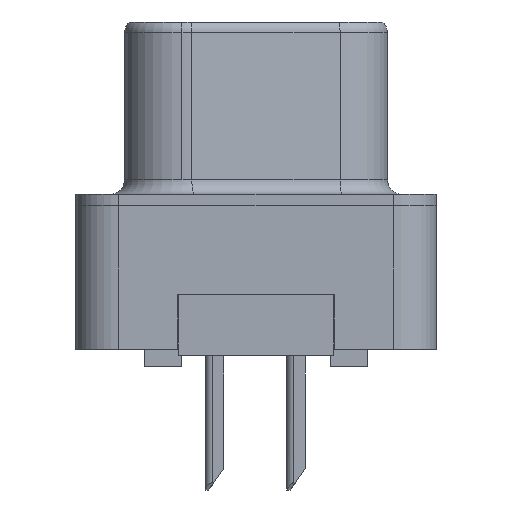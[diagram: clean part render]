
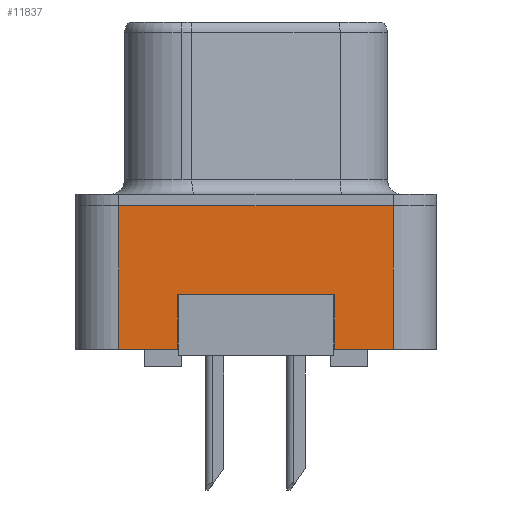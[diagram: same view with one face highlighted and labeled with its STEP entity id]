
A CAD part, left-side view. The second image highlights one B-rep face of the part: STEP entity #11837.
In plain terms, the highlighted planar face has unit normal (-1, 0, 0).
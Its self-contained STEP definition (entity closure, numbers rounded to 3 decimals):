
#8 = LINE ( 'NONE', #12915, #7780 ) ;
#268 = DIRECTION ( 'NONE',  ( 0., 0., 1. ) ) ;
#650 = LINE ( 'NONE', #9021, #14056 ) ;
#804 = CARTESIAN_POINT ( 'NONE',  ( -2.91, 2.75, -5. ) ) ;
#866 = VERTEX_POINT ( 'NONE', #6942 ) ;
#1035 = ORIENTED_EDGE ( 'NONE', *, *, #11643, .F. ) ;
#1530 = VECTOR ( 'NONE', #8417, 1000. ) ;
#1874 = DIRECTION ( 'NONE',  ( 0., -1., 0. ) ) ;
#2149 = ORIENTED_EDGE ( 'NONE', *, *, #11840, .T. ) ;
#3065 = DIRECTION ( 'NONE',  ( 0., 1., 0. ) ) ;
#3103 = VERTEX_POINT ( 'NONE', #804 ) ;
#3646 = CARTESIAN_POINT ( 'NONE',  ( -2.91, -4.775, -5. ) ) ;
#3878 = PLANE ( 'NONE',  #14046 ) ;
#3947 = EDGE_CURVE ( 'NONE', #15031, #7151, #7125, .T. ) ;
#4332 = EDGE_CURVE ( 'NONE', #7151, #10325, #8716, .T. ) ;
#4703 = DIRECTION ( 'NONE',  ( 0., 0., -1. ) ) ;
#4721 = VERTEX_POINT ( 'NONE', #8244 ) ;
#4814 = VECTOR ( 'NONE', #3065, 1000. ) ;
#4855 = DIRECTION ( 'NONE',  ( 0., 0., -1. ) ) ;
#4998 = ORIENTED_EDGE ( 'NONE', *, *, #14515, .F. ) ;
#5309 = VERTEX_POINT ( 'NONE', #13141 ) ;
#5919 = CARTESIAN_POINT ( 'NONE',  ( -2.91, 4.775, -5. ) ) ;
#5976 = ORIENTED_EDGE ( 'NONE', *, *, #3947, .T. ) ;
#6221 = DIRECTION ( 'NONE',  ( -1., 0., 0. ) ) ;
#6303 = VERTEX_POINT ( 'NONE', #8653 ) ;
#6375 = CARTESIAN_POINT ( 'NONE',  ( -2.91, -4.775, -5. ) ) ;
#6508 = CARTESIAN_POINT ( 'NONE',  ( -2.91, 2.75, -3.1 ) ) ;
#6942 = CARTESIAN_POINT ( 'NONE',  ( -2.91, 4.775, -5. ) ) ;
#7125 = LINE ( 'NONE', #11896, #13209 ) ;
#7151 = VERTEX_POINT ( 'NONE', #12938 ) ;
#7542 = DIRECTION ( 'NONE',  ( 0., -1., 0. ) ) ;
#7545 = FACE_OUTER_BOUND ( 'NONE', #11631, .T. ) ;
#7780 = VECTOR ( 'NONE', #4703, 1000. ) ;
#7811 = LINE ( 'NONE', #12593, #8017 ) ;
#8017 = VECTOR ( 'NONE', #1874, 1000. ) ;
#8244 = CARTESIAN_POINT ( 'NONE',  ( -2.91, -4.775, 0. ) ) ;
#8417 = DIRECTION ( 'NONE',  ( 0., 0., 1. ) ) ;
#8637 = CARTESIAN_POINT ( 'NONE',  ( -2.91, -2.75, -3.1 ) ) ;
#8653 = CARTESIAN_POINT ( 'NONE',  ( -2.91, 4.775, 0. ) ) ;
#8716 = LINE ( 'NONE', #3646, #9717 ) ;
#8791 = DIRECTION ( 'NONE',  ( 0., -1., 0. ) ) ;
#9021 = CARTESIAN_POINT ( 'NONE',  ( -2.91, -4.775, 0. ) ) ;
#9490 = ORIENTED_EDGE ( 'NONE', *, *, #13112, .F. ) ;
#9554 = ORIENTED_EDGE ( 'NONE', *, *, #10947, .T. ) ;
#9717 = VECTOR ( 'NONE', #7542, 1000. ) ;
#10325 = VERTEX_POINT ( 'NONE', #13328 ) ;
#10788 = VECTOR ( 'NONE', #11132, 1000. ) ;
#10849 = ORIENTED_EDGE ( 'NONE', *, *, #4332, .T. ) ;
#10947 = EDGE_CURVE ( 'NONE', #866, #3103, #7811, .T. ) ;
#11132 = DIRECTION ( 'NONE',  ( 0., 0., 1. ) ) ;
#11631 = EDGE_LOOP ( 'NONE', ( #5976, #10849, #2149, #13181, #1035, #9554, #9490, #4998 ) ) ;
#11643 = EDGE_CURVE ( 'NONE', #866, #6303, #11935, .T. ) ;
#11837 = ADVANCED_FACE ( 'NONE', ( #7545 ), #3878, .T. ) ;
#11840 = EDGE_CURVE ( 'NONE', #10325, #4721, #12325, .T. ) ;
#11896 = CARTESIAN_POINT ( 'NONE',  ( -2.91, -2.75, -3.1 ) ) ;
#11935 = LINE ( 'NONE', #5919, #1530 ) ;
#12165 = CARTESIAN_POINT ( 'NONE',  ( -2.91, -4.775, -5. ) ) ;
#12325 = LINE ( 'NONE', #6375, #10788 ) ;
#12593 = CARTESIAN_POINT ( 'NONE',  ( -2.91, -4.775, -5. ) ) ;
#12915 = CARTESIAN_POINT ( 'NONE',  ( -2.91, 2.75, -3.1 ) ) ;
#12938 = CARTESIAN_POINT ( 'NONE',  ( -2.91, -2.75, -5. ) ) ;
#13112 = EDGE_CURVE ( 'NONE', #5309, #3103, #8, .T. ) ;
#13141 = CARTESIAN_POINT ( 'NONE',  ( -2.91, 2.75, -3.1 ) ) ;
#13181 = ORIENTED_EDGE ( 'NONE', *, *, #13965, .F. ) ;
#13209 = VECTOR ( 'NONE', #4855, 1000. ) ;
#13328 = CARTESIAN_POINT ( 'NONE',  ( -2.91, -4.775, -5. ) ) ;
#13965 = EDGE_CURVE ( 'NONE', #6303, #4721, #650, .T. ) ;
#14046 = AXIS2_PLACEMENT_3D ( 'NONE', #12165, #6221, #268 ) ;
#14056 = VECTOR ( 'NONE', #8791, 1000. ) ;
#14515 = EDGE_CURVE ( 'NONE', #15031, #5309, #14955, .T. ) ;
#14955 = LINE ( 'NONE', #6508, #4814 ) ;
#15031 = VERTEX_POINT ( 'NONE', #8637 ) ;
